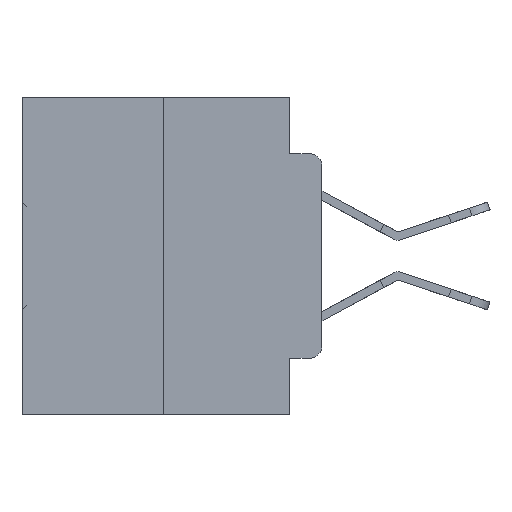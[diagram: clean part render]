
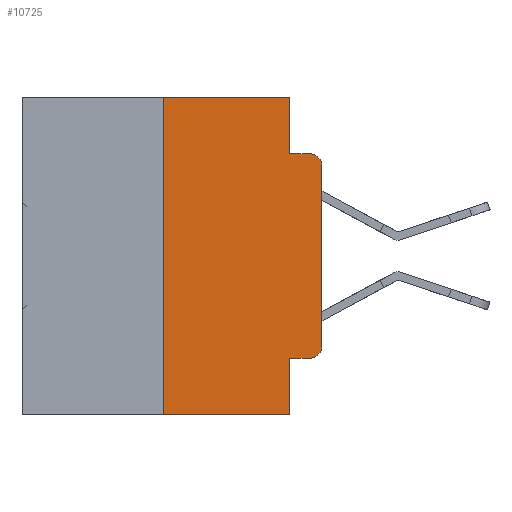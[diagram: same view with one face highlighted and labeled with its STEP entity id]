
A CAD part, left-side view. The second image highlights one B-rep face of the part: STEP entity #10725.
In plain terms, the highlighted planar face has unit normal (-1, 0, 0).
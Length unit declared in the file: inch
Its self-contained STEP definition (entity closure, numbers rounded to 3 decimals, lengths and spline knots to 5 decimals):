
#278 = DIRECTION ( 'NONE',  ( 0., 0., -1. ) ) ;
#1612 = VERTEX_POINT ( 'NONE', #2647 ) ;
#1622 = DIRECTION ( 'NONE',  ( 0., 0., -1. ) ) ;
#2003 = PLANE ( 'NONE',  #8558 ) ;
#2647 = CARTESIAN_POINT ( 'NONE',  ( 0., 0.25, -0.5 ) ) ;
#3508 = LINE ( 'NONE', #32133, #16950 ) ;
#3582 = DIRECTION ( 'NONE',  ( 0., -1., 0. ) ) ;
#3683 = CARTESIAN_POINT ( 'NONE',  ( 0., 0.02, -0.0885 ) ) ;
#3687 = CARTESIAN_POINT ( 'NONE',  ( 0., 0., -0.1085 ) ) ;
#4114 = EDGE_CURVE ( 'NONE', #1612, #5646, #33986, .T. ) ;
#4219 = CARTESIAN_POINT ( 'NONE',  ( 0., 0.051, -0.4115 ) ) ;
#4463 = VERTEX_POINT ( 'NONE', #4219 ) ;
#4642 = LINE ( 'NONE', #17207, #25032 ) ;
#5027 = VECTOR ( 'NONE', #9486, 39.37008 ) ;
#5371 = EDGE_LOOP ( 'NONE', ( #20633, #22287, #23944, #18588, #25601, #13210, #8567, #19011, #5657, #27669 ) ) ;
#5646 = VERTEX_POINT ( 'NONE', #14975 ) ;
#5657 = ORIENTED_EDGE ( 'NONE', *, *, #13305, .T. ) ;
#5878 = CARTESIAN_POINT ( 'NONE',  ( 0., 0., 0. ) ) ;
#6613 = DIRECTION ( 'NONE',  ( 0., -1., 0. ) ) ;
#7441 = FACE_OUTER_BOUND ( 'NONE', #5371, .T. ) ;
#7552 = VERTEX_POINT ( 'NONE', #9017 ) ;
#8068 = DIRECTION ( 'NONE',  ( -1., 0., 0. ) ) ;
#8090 = EDGE_CURVE ( 'NONE', #34006, #9834, #10349, .T. ) ;
#8161 = VERTEX_POINT ( 'NONE', #30090 ) ;
#8457 = VECTOR ( 'NONE', #1622, 39.37008 ) ;
#8558 = AXIS2_PLACEMENT_3D ( 'NONE', #15483, #26103, #10232 ) ;
#8567 = ORIENTED_EDGE ( 'NONE', *, *, #4114, .T. ) ;
#8734 = CARTESIAN_POINT ( 'NONE',  ( 0., 0.051, -0.0885 ) ) ;
#9017 = CARTESIAN_POINT ( 'NONE',  ( 0., 0.02, -0.4115 ) ) ;
#9486 = DIRECTION ( 'NONE',  ( 0., 0., 1. ) ) ;
#9834 = VERTEX_POINT ( 'NONE', #3683 ) ;
#10232 = DIRECTION ( 'NONE',  ( 0., 0., -1. ) ) ;
#10349 = LINE ( 'NONE', #8734, #31352 ) ;
#10725 = ADVANCED_FACE ( 'NONE', ( #7441 ), #2003, .F. ) ;
#10830 = CARTESIAN_POINT ( 'NONE',  ( 0., 0.051, -0.0885 ) ) ;
#11323 = VERTEX_POINT ( 'NONE', #31031 ) ;
#13042 = CIRCLE ( 'NONE', #30365, 0.02 ) ;
#13210 = ORIENTED_EDGE ( 'NONE', *, *, #29160, .F. ) ;
#13305 = EDGE_CURVE ( 'NONE', #4463, #7552, #22302, .T. ) ;
#13881 = AXIS2_PLACEMENT_3D ( 'NONE', #23987, #8068, #26635 ) ;
#14829 = EDGE_CURVE ( 'NONE', #11323, #34006, #15583, .T. ) ;
#14975 = CARTESIAN_POINT ( 'NONE',  ( 0., 0.051, -0.5 ) ) ;
#15411 = VERTEX_POINT ( 'NONE', #29579 ) ;
#15451 = CARTESIAN_POINT ( 'NONE',  ( 0., 0.02, -0.3915 ) ) ;
#15483 = CARTESIAN_POINT ( 'NONE',  ( 0., 0.473, 0. ) ) ;
#15583 = LINE ( 'NONE', #17790, #8457 ) ;
#15600 = EDGE_CURVE ( 'NONE', #15411, #11323, #4642, .T. ) ;
#15789 = EDGE_CURVE ( 'NONE', #7552, #8161, #13042, .T. ) ;
#15944 = EDGE_CURVE ( 'NONE', #18081, #9834, #30944, .T. ) ;
#16950 = VECTOR ( 'NONE', #278, 39.37008 ) ;
#16965 = CARTESIAN_POINT ( 'NONE',  ( 0., 0.051, -0.4115 ) ) ;
#17207 = CARTESIAN_POINT ( 'NONE',  ( 0., 0.473, 0. ) ) ;
#17790 = CARTESIAN_POINT ( 'NONE',  ( 0., 0.051, 0. ) ) ;
#18081 = VERTEX_POINT ( 'NONE', #3687 ) ;
#18116 = DIRECTION ( 'NONE',  ( 0., 0., -1. ) ) ;
#18588 = ORIENTED_EDGE ( 'NONE', *, *, #14829, .F. ) ;
#19011 = ORIENTED_EDGE ( 'NONE', *, *, #32080, .F. ) ;
#19200 = LINE ( 'NONE', #5878, #32247 ) ;
#19820 = VECTOR ( 'NONE', #3582, 39.37008 ) ;
#20633 = ORIENTED_EDGE ( 'NONE', *, *, #27194, .T. ) ;
#20977 = VECTOR ( 'NONE', #6613, 39.37008 ) ;
#22287 = ORIENTED_EDGE ( 'NONE', *, *, #15944, .T. ) ;
#22302 = LINE ( 'NONE', #16965, #19820 ) ;
#23944 = ORIENTED_EDGE ( 'NONE', *, *, #8090, .F. ) ;
#23987 = CARTESIAN_POINT ( 'NONE',  ( 0., 0.02, -0.1085 ) ) ;
#25032 = VECTOR ( 'NONE', #30259, 39.37008 ) ;
#25601 = ORIENTED_EDGE ( 'NONE', *, *, #15600, .F. ) ;
#26103 = DIRECTION ( 'NONE',  ( 1., 0., 0. ) ) ;
#26635 = DIRECTION ( 'NONE',  ( 0., 0., -1. ) ) ;
#27124 = DIRECTION ( 'NONE',  ( 0., 0., 1. ) ) ;
#27194 = EDGE_CURVE ( 'NONE', #8161, #18081, #19200, .T. ) ;
#27669 = ORIENTED_EDGE ( 'NONE', *, *, #15789, .T. ) ;
#29160 = EDGE_CURVE ( 'NONE', #1612, #15411, #33092, .T. ) ;
#29579 = CARTESIAN_POINT ( 'NONE',  ( 0., 0.25, 0. ) ) ;
#29866 = DIRECTION ( 'NONE',  ( 0., -1., 0. ) ) ;
#30031 = CARTESIAN_POINT ( 'NONE',  ( 0., 0.473, -0.5 ) ) ;
#30090 = CARTESIAN_POINT ( 'NONE',  ( 0., 0., -0.3915 ) ) ;
#30259 = DIRECTION ( 'NONE',  ( 0., -1., 0. ) ) ;
#30365 = AXIS2_PLACEMENT_3D ( 'NONE', #15451, #33730, #18116 ) ;
#30590 = CARTESIAN_POINT ( 'NONE',  ( 0., 0.25, 0. ) ) ;
#30944 = CIRCLE ( 'NONE', #13881, 0.02 ) ;
#31031 = CARTESIAN_POINT ( 'NONE',  ( 0., 0.051, 0. ) ) ;
#31352 = VECTOR ( 'NONE', #29866, 39.37008 ) ;
#32080 = EDGE_CURVE ( 'NONE', #4463, #5646, #3508, .T. ) ;
#32133 = CARTESIAN_POINT ( 'NONE',  ( 0., 0.051, 0. ) ) ;
#32247 = VECTOR ( 'NONE', #27124, 39.37008 ) ;
#33092 = LINE ( 'NONE', #30590, #5027 ) ;
#33730 = DIRECTION ( 'NONE',  ( -1., 0., 0. ) ) ;
#33986 = LINE ( 'NONE', #30031, #20977 ) ;
#34006 = VERTEX_POINT ( 'NONE', #10830 ) ;
